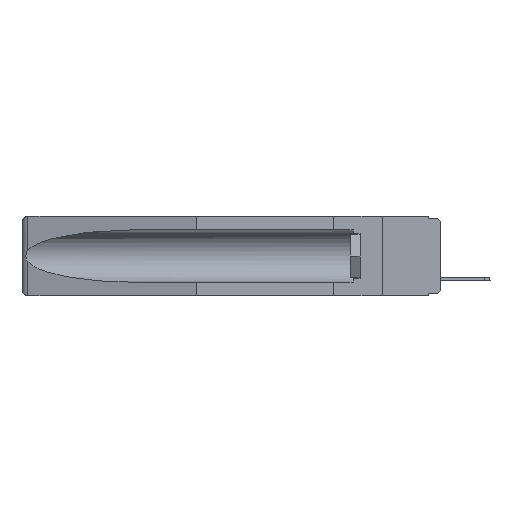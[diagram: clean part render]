
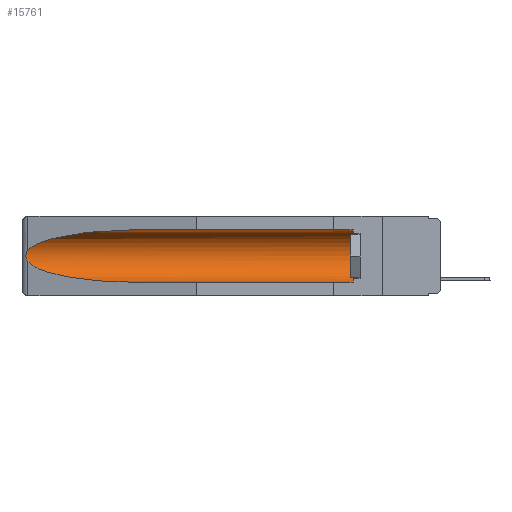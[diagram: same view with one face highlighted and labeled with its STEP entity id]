
A CAD part, left-side view. The second image highlights one B-rep face of the part: STEP entity #15761.
In plain terms, the highlighted cylindrical face has radius 2.857 mm (diameter 5.715 mm), a partial arc.
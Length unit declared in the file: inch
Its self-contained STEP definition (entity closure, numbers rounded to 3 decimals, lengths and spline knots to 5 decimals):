
#136 = ORIENTED_EDGE ( 'NONE', *, *, #11255, .T. ) ;
#180 = CARTESIAN_POINT ( 'NONE',  ( 0.155, -0.30754, -0.284 ) ) ;
#273 = DIRECTION ( 'NONE',  ( 0., 1., 0. ) ) ;
#511 = CARTESIAN_POINT ( 'NONE',  ( 0.26537, 1.52718, -0.14972 ) ) ;
#704 = CARTESIAN_POINT ( 'NONE',  ( 0.155, 1.07973, -0.284 ) ) ;
#743 = CARTESIAN_POINT ( 'NONE',  ( 0.25451, 1.48313, -0.09465 ) ) ;
#1801 = DIRECTION ( 'NONE',  ( 0., -1., 0. ) ) ;
#1894 = CARTESIAN_POINT ( 'NONE',  ( 0.155, 0.126, -0.1715 ) ) ;
#2053 = ORIENTED_EDGE ( 'NONE', *, *, #2899, .F. ) ;
#2191 = CARTESIAN_POINT ( 'NONE',  ( 0.26537, 1.52718, -0.14972 ) ) ;
#2899 = EDGE_CURVE ( 'NONE', #13882, #12118, #13797, .T. ) ;
#3356 =( BOUNDED_CURVE ( )  B_SPLINE_CURVE ( 3, ( #6353, #14620, #743, #2191 ),
 .UNSPECIFIED., .F., .F. ) 
 B_SPLINE_CURVE_WITH_KNOTS ( ( 4, 4 ),
 ( 4.71239, 6.08839 ),
 .UNSPECIFIED. ) 
 CURVE ( )  GEOMETRIC_REPRESENTATION_ITEM ( )  RATIONAL_B_SPLINE_CURVE ( ( 1., 0.848, 0.848, 1. ) ) 
 REPRESENTATION_ITEM ( '' )  );
#3483 = CARTESIAN_POINT ( 'NONE',  ( 0.155, 0.126, -0.284 ) ) ;
#3591 = CARTESIAN_POINT ( 'NONE',  ( 0.155, -0.30754, -0.1715 ) ) ;
#3735 = CARTESIAN_POINT ( 'NONE',  ( 0.2675, 1.53308, -0.16763 ) ) ;
#3804 = EDGE_LOOP ( 'NONE', ( #136, #17619, #7706, #2053, #11587, #17851 ) ) ;
#4271 = EDGE_CURVE ( 'NONE', #13882, #17391, #6582, .T. ) ;
#4512 = DIRECTION ( 'NONE',  ( 0., 0., 1. ) ) ;
#4678 = DIRECTION ( 'NONE',  ( 0., 1., 0. ) ) ;
#4864 = DIRECTION ( 'NONE',  ( 0., 0., 1. ) ) ;
#4923 = CARTESIAN_POINT ( 'NONE',  ( 0.26597, 1.52961, -0.15275 ) ) ;
#5157 = B_SPLINE_CURVE_WITH_KNOTS ( 'NONE', 3,
 ( #13458, #4923, #7926, #17424, #3735, #9278, #14807, #17600, #6638, #14976 ),
 .UNSPECIFIED., .F., .F.,
 ( 4, 2, 2, 2, 4 ),
 ( 0., 0.00029, 0.00058, 0.00087, 0.00117 ),
 .UNSPECIFIED. ) ;
#6353 = CARTESIAN_POINT ( 'NONE',  ( 0.155, 1.07973, -0.059 ) ) ;
#6582 = CIRCLE ( 'NONE', #10640, 0.1125 ) ;
#6638 = CARTESIAN_POINT ( 'NONE',  ( 0.26597, 1.5296, -0.19026 ) ) ;
#7227 = EDGE_CURVE ( 'NONE', #9646, #17345, #5157, .T. ) ;
#7660 = CARTESIAN_POINT ( 'NONE',  ( 0.155, 0.126, -0.059 ) ) ;
#7706 = ORIENTED_EDGE ( 'NONE', *, *, #8961, .T. ) ;
#7926 = CARTESIAN_POINT ( 'NONE',  ( 0.26654, 1.53092, -0.15636 ) ) ;
#7998 = CARTESIAN_POINT ( 'NONE',  ( 0.26537, 1.52718, -0.19328 ) ) ;
#8084 = CARTESIAN_POINT ( 'NONE',  ( 0.155, 1.07973, -0.284 ) ) ;
#8236 = LINE ( 'NONE', #12655, #13473 ) ;
#8266 = VECTOR ( 'NONE', #273, 39.37008 ) ;
#8961 = EDGE_CURVE ( 'NONE', #17345, #12118, #12053, .T. ) ;
#9278 = CARTESIAN_POINT ( 'NONE',  ( 0.2675, 1.53308, -0.17534 ) ) ;
#9646 = VERTEX_POINT ( 'NONE', #511 ) ;
#10476 = CARTESIAN_POINT ( 'NONE',  ( 0.26537, 1.52718, -0.19328 ) ) ;
#10640 = AXIS2_PLACEMENT_3D ( 'NONE', #1894, #1801, #4512 ) ;
#11255 = EDGE_CURVE ( 'NONE', #16709, #9646, #3356, .T. ) ;
#11587 = ORIENTED_EDGE ( 'NONE', *, *, #4271, .T. ) ;
#11758 = FACE_OUTER_BOUND ( 'NONE', #3804, .T. ) ;
#12033 = EDGE_CURVE ( 'NONE', #17391, #16709, #8236, .T. ) ;
#12053 =( BOUNDED_CURVE ( )  B_SPLINE_CURVE ( 3, ( #7998, #17671, #14964, #8084 ),
 .UNSPECIFIED., .F., .T. ) 
 B_SPLINE_CURVE_WITH_KNOTS ( ( 4, 4 ),
 ( 0.1948, 1.5708 ),
 .UNSPECIFIED. ) 
 CURVE ( )  GEOMETRIC_REPRESENTATION_ITEM ( )  RATIONAL_B_SPLINE_CURVE ( ( 1., 0.848, 0.848, 1. ) ) 
 REPRESENTATION_ITEM ( '' )  );
#12118 = VERTEX_POINT ( 'NONE', #704 ) ;
#12143 = CARTESIAN_POINT ( 'NONE',  ( 0.155, 1.07973, -0.059 ) ) ;
#12314 = DIRECTION ( 'NONE',  ( 0., 1., 0. ) ) ;
#12655 = CARTESIAN_POINT ( 'NONE',  ( 0.155, -0.30754, -0.059 ) ) ;
#13458 = CARTESIAN_POINT ( 'NONE',  ( 0.26537, 1.52718, -0.14972 ) ) ;
#13473 = VECTOR ( 'NONE', #12314, 39.37008 ) ;
#13601 = AXIS2_PLACEMENT_3D ( 'NONE', #3591, #4678, #4864 ) ;
#13797 = LINE ( 'NONE', #180, #8266 ) ;
#13882 = VERTEX_POINT ( 'NONE', #3483 ) ;
#14620 = CARTESIAN_POINT ( 'NONE',  ( 0.21114, 1.30732, -0.059 ) ) ;
#14807 = CARTESIAN_POINT ( 'NONE',  ( 0.2673, 1.53269, -0.17917 ) ) ;
#14964 = CARTESIAN_POINT ( 'NONE',  ( 0.21114, 1.30732, -0.284 ) ) ;
#14976 = CARTESIAN_POINT ( 'NONE',  ( 0.26537, 1.52718, -0.19328 ) ) ;
#15761 = ADVANCED_FACE ( 'NONE', ( #11758 ), #17266, .F. ) ;
#16709 = VERTEX_POINT ( 'NONE', #12143 ) ;
#17266 = CYLINDRICAL_SURFACE ( 'NONE', #13601, 0.1125 ) ;
#17345 = VERTEX_POINT ( 'NONE', #10476 ) ;
#17391 = VERTEX_POINT ( 'NONE', #7660 ) ;
#17424 = CARTESIAN_POINT ( 'NONE',  ( 0.2673, 1.5327, -0.16383 ) ) ;
#17600 = CARTESIAN_POINT ( 'NONE',  ( 0.26655, 1.53094, -0.18657 ) ) ;
#17619 = ORIENTED_EDGE ( 'NONE', *, *, #7227, .T. ) ;
#17671 = CARTESIAN_POINT ( 'NONE',  ( 0.25451, 1.48313, -0.24835 ) ) ;
#17851 = ORIENTED_EDGE ( 'NONE', *, *, #12033, .T. ) ;
